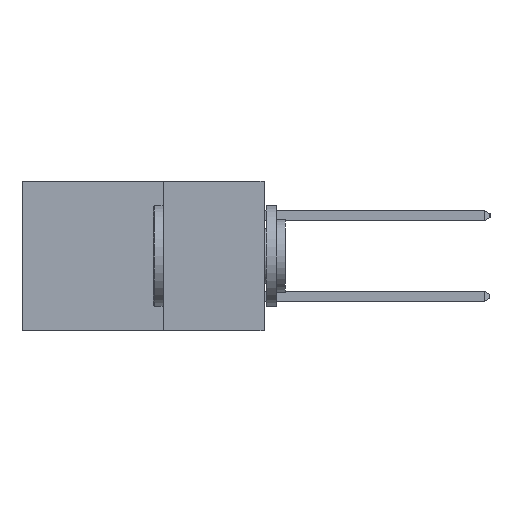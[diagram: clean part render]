
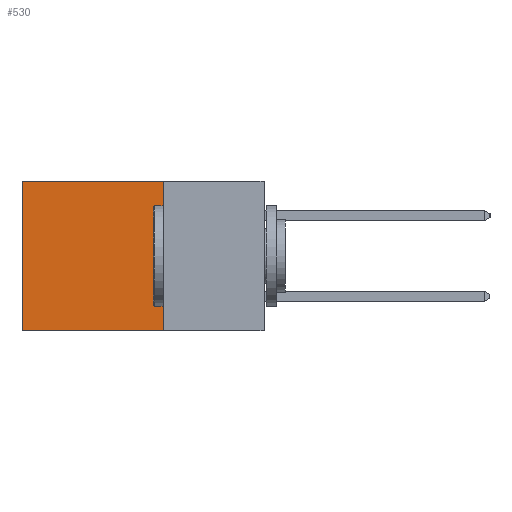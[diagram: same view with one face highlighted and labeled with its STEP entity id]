
A CAD part, left-side view. The second image highlights one B-rep face of the part: STEP entity #530.
In plain terms, the highlighted planar face has unit normal (-1, 0, 0).
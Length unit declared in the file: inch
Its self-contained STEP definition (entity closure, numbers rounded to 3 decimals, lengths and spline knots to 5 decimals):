
#289 = VERTEX_POINT ( 'NONE', #11916 ) ;
#317 = VECTOR ( 'NONE', #4280, 39.37008 ) ;
#530 = ADVANCED_FACE ( 'NONE', ( #8700 ), #4823, .F. ) ;
#601 = CARTESIAN_POINT ( 'NONE',  ( 0.2615, 0.6, 0. ) ) ;
#988 = LINE ( 'NONE', #8875, #11440 ) ;
#1789 = VERTEX_POINT ( 'NONE', #3626 ) ;
#2834 = EDGE_CURVE ( 'NONE', #8264, #289, #988, .T. ) ;
#3626 = CARTESIAN_POINT ( 'NONE',  ( 0.2615, 0.25, 0. ) ) ;
#3803 = LINE ( 'NONE', #4582, #7302 ) ;
#3823 = CARTESIAN_POINT ( 'NONE',  ( 0.2615, 0.25, -0.37 ) ) ;
#4280 = DIRECTION ( 'NONE',  ( 0., 0., -1. ) ) ;
#4582 = CARTESIAN_POINT ( 'NONE',  ( 0.2615, 0.25, 0. ) ) ;
#4636 = DIRECTION ( 'NONE',  ( 0., 0., -1. ) ) ;
#4823 = PLANE ( 'NONE',  #6916 ) ;
#5233 = LINE ( 'NONE', #5308, #317 ) ;
#5308 = CARTESIAN_POINT ( 'NONE',  ( 0.2615, 0.25, -0.37 ) ) ;
#5577 = DIRECTION ( 'NONE',  ( 0., 1., 0. ) ) ;
#5735 = DIRECTION ( 'NONE',  ( 0., 1., 0. ) ) ;
#6685 = VECTOR ( 'NONE', #5577, 39.37008 ) ;
#6881 = ORIENTED_EDGE ( 'NONE', *, *, #11315, .T. ) ;
#6916 = AXIS2_PLACEMENT_3D ( 'NONE', #8831, #12774, #4636 ) ;
#7302 = VECTOR ( 'NONE', #5735, 39.37008 ) ;
#7353 = EDGE_CURVE ( 'NONE', #1789, #12806, #5233, .T. ) ;
#7793 = DIRECTION ( 'NONE',  ( 0., 0., -1. ) ) ;
#8264 = VERTEX_POINT ( 'NONE', #601 ) ;
#8631 = CARTESIAN_POINT ( 'NONE',  ( 0.2615, 0.25, -0.37 ) ) ;
#8700 = FACE_OUTER_BOUND ( 'NONE', #10079, .T. ) ;
#8831 = CARTESIAN_POINT ( 'NONE',  ( 0.2615, 0.25, -0.37 ) ) ;
#8872 = ORIENTED_EDGE ( 'NONE', *, *, #2834, .T. ) ;
#8875 = CARTESIAN_POINT ( 'NONE',  ( 0.2615, 0.6, -0.37 ) ) ;
#10079 = EDGE_LOOP ( 'NONE', ( #8872, #12279, #12488, #6881 ) ) ;
#10550 = LINE ( 'NONE', #8631, #6685 ) ;
#11315 = EDGE_CURVE ( 'NONE', #1789, #8264, #3803, .T. ) ;
#11440 = VECTOR ( 'NONE', #7793, 39.37008 ) ;
#11916 = CARTESIAN_POINT ( 'NONE',  ( 0.2615, 0.6, -0.37 ) ) ;
#12082 = EDGE_CURVE ( 'NONE', #12806, #289, #10550, .T. ) ;
#12279 = ORIENTED_EDGE ( 'NONE', *, *, #12082, .F. ) ;
#12488 = ORIENTED_EDGE ( 'NONE', *, *, #7353, .F. ) ;
#12774 = DIRECTION ( 'NONE',  ( 1., 0., 0. ) ) ;
#12806 = VERTEX_POINT ( 'NONE', #3823 ) ;
